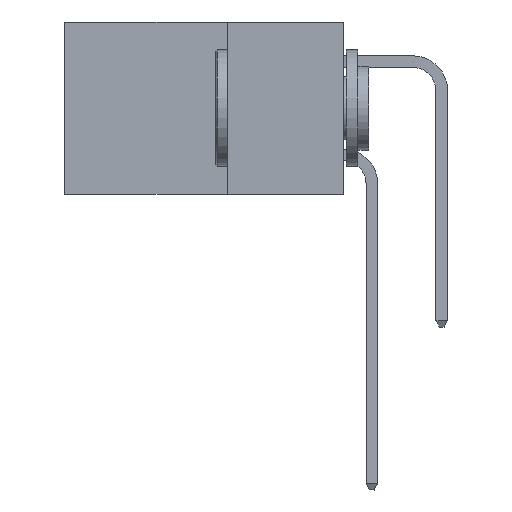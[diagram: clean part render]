
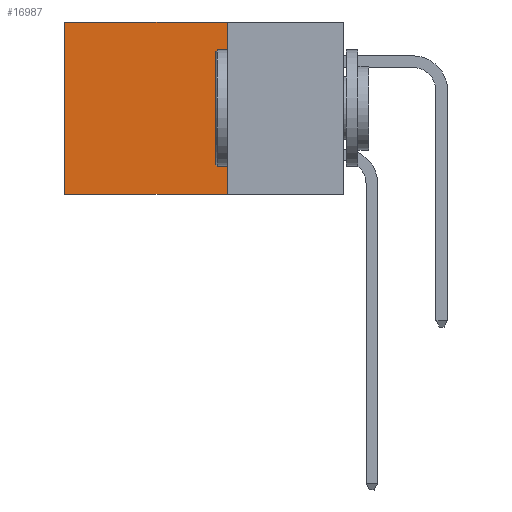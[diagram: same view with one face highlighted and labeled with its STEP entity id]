
A CAD part, left-side view. The second image highlights one B-rep face of the part: STEP entity #16987.
In plain terms, the highlighted planar face has unit normal (-1, 0, 0).
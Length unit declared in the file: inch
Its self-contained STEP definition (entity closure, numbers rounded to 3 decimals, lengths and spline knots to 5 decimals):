
#1312 = EDGE_CURVE ( 'NONE', #6637, #9186, #3555, .T. ) ;
#2016 = ORIENTED_EDGE ( 'NONE', *, *, #1312, .F. ) ;
#2233 = CARTESIAN_POINT ( 'NONE',  ( 0.298, 0.25, 0. ) ) ;
#2280 = LINE ( 'NONE', #21235, #13257 ) ;
#3171 = CARTESIAN_POINT ( 'NONE',  ( 0.298, 0.6, 0. ) ) ;
#3555 = LINE ( 'NONE', #20049, #8562 ) ;
#5962 = PLANE ( 'NONE',  #17170 ) ;
#6088 = ORIENTED_EDGE ( 'NONE', *, *, #16259, .T. ) ;
#6637 = VERTEX_POINT ( 'NONE', #11639 ) ;
#7934 = DIRECTION ( 'NONE',  ( 0., 1., 0. ) ) ;
#8562 = VECTOR ( 'NONE', #8918, 39.37008 ) ;
#8918 = DIRECTION ( 'NONE',  ( 0., 1., 0. ) ) ;
#9010 = VECTOR ( 'NONE', #7934, 39.37008 ) ;
#9082 = CARTESIAN_POINT ( 'NONE',  ( 0.298, 0.6, 0. ) ) ;
#9186 = VERTEX_POINT ( 'NONE', #9735 ) ;
#9532 = VERTEX_POINT ( 'NONE', #3171 ) ;
#9694 = DIRECTION ( 'NONE',  ( 1., 0., 0. ) ) ;
#9735 = CARTESIAN_POINT ( 'NONE',  ( 0.298, 0.6, -0.37 ) ) ;
#11639 = CARTESIAN_POINT ( 'NONE',  ( 0.298, 0.25, -0.37 ) ) ;
#11949 = VERTEX_POINT ( 'NONE', #15341 ) ;
#12580 = DIRECTION ( 'NONE',  ( 0., 0., -1. ) ) ;
#13257 = VECTOR ( 'NONE', #12580, 39.37008 ) ;
#13601 = ORIENTED_EDGE ( 'NONE', *, *, #18659, .T. ) ;
#14149 = VECTOR ( 'NONE', #21433, 39.37008 ) ;
#15341 = CARTESIAN_POINT ( 'NONE',  ( 0.298, 0.25, 0. ) ) ;
#15404 = LINE ( 'NONE', #2233, #9010 ) ;
#16259 = EDGE_CURVE ( 'NONE', #9532, #9186, #18220, .T. ) ;
#16707 = CARTESIAN_POINT ( 'NONE',  ( 0.298, 0.25, 0. ) ) ;
#16816 = FACE_OUTER_BOUND ( 'NONE', #19623, .T. ) ;
#16987 = ADVANCED_FACE ( 'NONE', ( #16816 ), #5962, .F. ) ;
#17170 = AXIS2_PLACEMENT_3D ( 'NONE', #16707, #9694, #22017 ) ;
#17416 = EDGE_CURVE ( 'NONE', #11949, #6637, #2280, .T. ) ;
#18220 = LINE ( 'NONE', #9082, #14149 ) ;
#18659 = EDGE_CURVE ( 'NONE', #11949, #9532, #15404, .T. ) ;
#19623 = EDGE_LOOP ( 'NONE', ( #6088, #2016, #21664, #13601 ) ) ;
#20049 = CARTESIAN_POINT ( 'NONE',  ( 0.298, 0.25, -0.37 ) ) ;
#21235 = CARTESIAN_POINT ( 'NONE',  ( 0.298, 0.25, 0. ) ) ;
#21433 = DIRECTION ( 'NONE',  ( 0., 0., -1. ) ) ;
#21664 = ORIENTED_EDGE ( 'NONE', *, *, #17416, .F. ) ;
#22017 = DIRECTION ( 'NONE',  ( 0., 0., -1. ) ) ;
